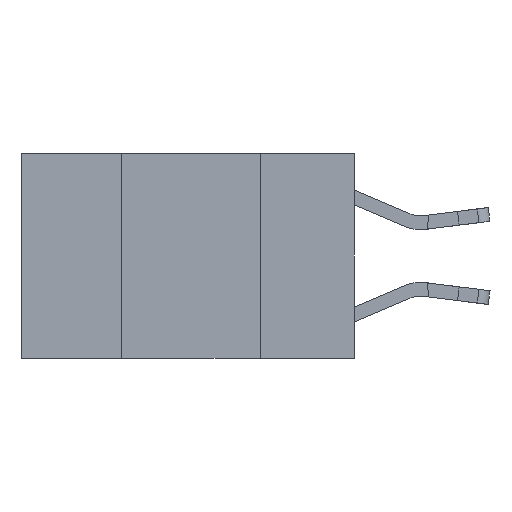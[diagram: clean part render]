
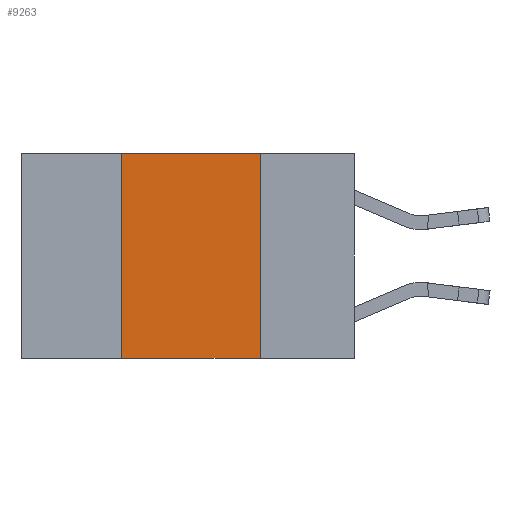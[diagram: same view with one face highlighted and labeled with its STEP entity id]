
A CAD part, left-side view. The second image highlights one B-rep face of the part: STEP entity #9263.
In plain terms, the highlighted planar face has unit normal (-1, 0, 0).
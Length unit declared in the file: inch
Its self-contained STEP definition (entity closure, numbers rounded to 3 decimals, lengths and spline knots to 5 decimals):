
#83 = CARTESIAN_POINT ( 'NONE',  ( 0., 0.42, 0. ) ) ;
#258 = CARTESIAN_POINT ( 'NONE',  ( 0., 0.17, 0. ) ) ;
#504 = EDGE_CURVE ( 'NONE', #13001, #1408, #11581, .T. ) ;
#508 = DIRECTION ( 'NONE',  ( 0., 0., -1. ) ) ;
#1408 = VERTEX_POINT ( 'NONE', #5719 ) ;
#2438 = VERTEX_POINT ( 'NONE', #258 ) ;
#2756 = ORIENTED_EDGE ( 'NONE', *, *, #504, .T. ) ;
#3161 = VECTOR ( 'NONE', #5080, 39.37008 ) ;
#3690 = LINE ( 'NONE', #9542, #8970 ) ;
#3813 = EDGE_CURVE ( 'NONE', #4663, #2438, #3690, .T. ) ;
#3955 = CARTESIAN_POINT ( 'NONE',  ( 0., 0.6, -0.37 ) ) ;
#4569 = PLANE ( 'NONE',  #7508 ) ;
#4663 = VERTEX_POINT ( 'NONE', #9561 ) ;
#5080 = DIRECTION ( 'NONE',  ( 0., -1., 0. ) ) ;
#5258 = DIRECTION ( 'NONE',  ( 0., 0., 1. ) ) ;
#5645 = DIRECTION ( 'NONE',  ( 1., 0., 0. ) ) ;
#5719 = CARTESIAN_POINT ( 'NONE',  ( 0., 0.17, -0.37 ) ) ;
#5956 = CARTESIAN_POINT ( 'NONE',  ( 0., 0.42, -0.37 ) ) ;
#7100 = LINE ( 'NONE', #7798, #9579 ) ;
#7470 = DIRECTION ( 'NONE',  ( 0., -1., 0. ) ) ;
#7508 = AXIS2_PLACEMENT_3D ( 'NONE', #11902, #5645, #12869 ) ;
#7614 = FACE_OUTER_BOUND ( 'NONE', #11937, .T. ) ;
#7798 = CARTESIAN_POINT ( 'NONE',  ( 0., 0.17, 0. ) ) ;
#8027 = EDGE_CURVE ( 'NONE', #2438, #1408, #7100, .T. ) ;
#8970 = VECTOR ( 'NONE', #7470, 39.37008 ) ;
#9123 = EDGE_CURVE ( 'NONE', #13001, #4663, #12606, .T. ) ;
#9263 = ADVANCED_FACE ( 'NONE', ( #7614 ), #4569, .F. ) ;
#9542 = CARTESIAN_POINT ( 'NONE',  ( 0., 0.6, 0. ) ) ;
#9561 = CARTESIAN_POINT ( 'NONE',  ( 0., 0.42, 0. ) ) ;
#9579 = VECTOR ( 'NONE', #508, 39.37008 ) ;
#9931 = VECTOR ( 'NONE', #5258, 39.37008 ) ;
#10863 = ORIENTED_EDGE ( 'NONE', *, *, #9123, .F. ) ;
#11581 = LINE ( 'NONE', #3955, #3161 ) ;
#11902 = CARTESIAN_POINT ( 'NONE',  ( 0., 0.6, 0. ) ) ;
#11937 = EDGE_LOOP ( 'NONE', ( #12860, #13190, #10863, #2756 ) ) ;
#12606 = LINE ( 'NONE', #83, #9931 ) ;
#12860 = ORIENTED_EDGE ( 'NONE', *, *, #8027, .F. ) ;
#12869 = DIRECTION ( 'NONE',  ( 0., 0., -1. ) ) ;
#13001 = VERTEX_POINT ( 'NONE', #5956 ) ;
#13190 = ORIENTED_EDGE ( 'NONE', *, *, #3813, .F. ) ;
